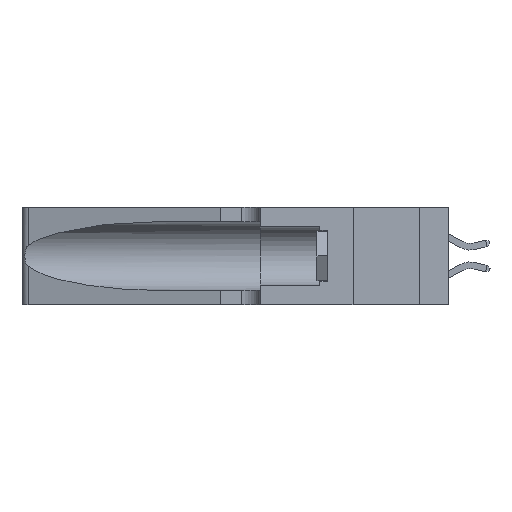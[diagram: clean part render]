
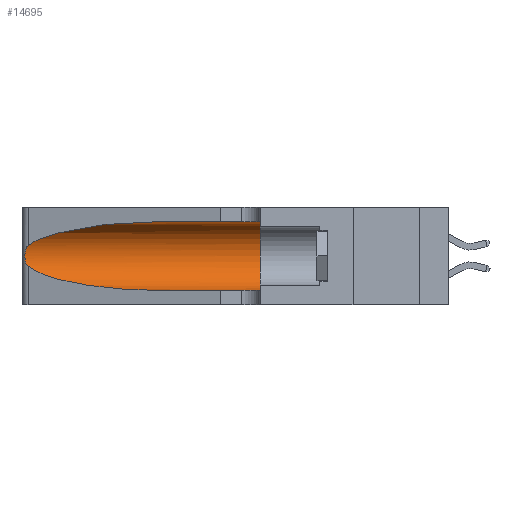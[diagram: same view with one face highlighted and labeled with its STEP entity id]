
A CAD part, left-side view. The second image highlights one B-rep face of the part: STEP entity #14695.
In plain terms, the highlighted cylindrical face has radius 3.308 mm (diameter 6.617 mm), a partial arc.
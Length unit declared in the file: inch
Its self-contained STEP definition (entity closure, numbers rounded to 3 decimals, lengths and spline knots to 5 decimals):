
#63 = VERTEX_POINT ( 'NONE', #3410 ) ;
#274 = CARTESIAN_POINT ( 'NONE',  ( 0.25789, 1.23486, 0.15765 ) ) ;
#662 = CARTESIAN_POINT ( 'NONE',  ( 0.2373, 1.15595, 0.08982 ) ) ;
#737 = CARTESIAN_POINT ( 'NONE',  ( 0.25487, 1.22718, 0.14631 ) ) ;
#1788 = CARTESIAN_POINT ( 'NONE',  ( 0.25487, 1.22718, 0.22369 ) ) ;
#1856 = CARTESIAN_POINT ( 'NONE',  ( 0.25555, 1.22993, 0.14849 ) ) ;
#2571 =( BOUNDED_CURVE ( )  B_SPLINE_CURVE ( 3, ( #16395, #17881, #8859, #19419 ),
 .UNSPECIFIED., .F., .F. ) 
 B_SPLINE_CURVE_WITH_KNOTS ( ( 4, 4 ),
 ( 1.5708, 2.84003 ),
 .UNSPECIFIED. ) 
 CURVE ( )  GEOMETRIC_REPRESENTATION_ITEM ( )  RATIONAL_B_SPLINE_CURVE ( ( 1., 0.87, 0.87, 1. ) ) 
 REPRESENTATION_ITEM ( '' )  );
#3218 = B_SPLINE_CURVE_WITH_KNOTS ( 'NONE', 3,
 ( #1788, #11126, #14113, #5010, #15631, #6554, #17138, #8082, #18642, #9629, #274, #11193, #1856, #12697 ),
 .UNSPECIFIED., .F., .F.,
 ( 4, 2, 2, 2, 2, 2, 4 ),
 ( 0., 0.00027, 0.00053, 0.00107, 0.0016, 0.00187, 0.00214 ),
 .UNSPECIFIED. ) ;
#3234 = CARTESIAN_POINT ( 'NONE',  ( 0.25487, 1.22718, 0.22369 ) ) ;
#3410 = CARTESIAN_POINT ( 'NONE',  ( 0.1305, 0.35, 0.31525 ) ) ;
#3639 = DIRECTION ( 'NONE',  ( 0., -1., 0. ) ) ;
#4037 = ORIENTED_EDGE ( 'NONE', *, *, #7615, .T. ) ;
#4151 =( BOUNDED_CURVE ( )  B_SPLINE_CURVE ( 3, ( #737, #662, #8533, #11639 ),
 .UNSPECIFIED., .F., .F. ) 
 B_SPLINE_CURVE_WITH_KNOTS ( ( 4, 4 ),
 ( 3.44316, 4.71239 ),
 .UNSPECIFIED. ) 
 CURVE ( )  GEOMETRIC_REPRESENTATION_ITEM ( )  RATIONAL_B_SPLINE_CURVE ( ( 1., 0.87, 0.87, 1. ) ) 
 REPRESENTATION_ITEM ( '' )  );
#4871 = LINE ( 'NONE', #17054, #16971 ) ;
#4933 = ORIENTED_EDGE ( 'NONE', *, *, #10686, .T. ) ;
#5001 = VERTEX_POINT ( 'NONE', #3234 ) ;
#5006 = VERTEX_POINT ( 'NONE', #16998 ) ;
#5010 = CARTESIAN_POINT ( 'NONE',  ( 0.25787, 1.23484, 0.2124 ) ) ;
#5095 = ORIENTED_EDGE ( 'NONE', *, *, #9715, .T. ) ;
#5724 = CARTESIAN_POINT ( 'NONE',  ( 0.1305, 0.35, 0.05475 ) ) ;
#5844 = AXIS2_PLACEMENT_3D ( 'NONE', #5921, #19493, #16521 ) ;
#5905 = ORIENTED_EDGE ( 'NONE', *, *, #11328, .F. ) ;
#5921 = CARTESIAN_POINT ( 'NONE',  ( 0.1305, 1.61858, 0.185 ) ) ;
#6327 = EDGE_LOOP ( 'NONE', ( #4933, #5095, #4037, #11713, #5905, #15191 ) ) ;
#6554 = CARTESIAN_POINT ( 'NONE',  ( 0.26018, 1.23835, 0.19895 ) ) ;
#6776 = CARTESIAN_POINT ( 'NONE',  ( 0.1305, 1.61858, 0.05475 ) ) ;
#6804 = CARTESIAN_POINT ( 'NONE',  ( 0.1305, 0.72297, 0.05475 ) ) ;
#6993 = CIRCLE ( 'NONE', #10850, 0.13025 ) ;
#7615 = EDGE_CURVE ( 'NONE', #13913, #9398, #4151, .T. ) ;
#7861 = CYLINDRICAL_SURFACE ( 'NONE', #5844, 0.13025 ) ;
#7997 = DIRECTION ( 'NONE',  ( 0., -1., 0. ) ) ;
#8082 = CARTESIAN_POINT ( 'NONE',  ( 0.26075, 1.23896, 0.178 ) ) ;
#8176 = EDGE_CURVE ( 'NONE', #9398, #10665, #16344, .T. ) ;
#8533 = CARTESIAN_POINT ( 'NONE',  ( 0.18966, 0.96281, 0.05475 ) ) ;
#8696 = CARTESIAN_POINT ( 'NONE',  ( 0.25487, 1.22718, 0.14631 ) ) ;
#8859 = CARTESIAN_POINT ( 'NONE',  ( 0.2373, 1.15595, 0.28018 ) ) ;
#8977 = CARTESIAN_POINT ( 'NONE',  ( 0.1305, 0.35, 0.185 ) ) ;
#9398 = VERTEX_POINT ( 'NONE', #6804 ) ;
#9629 = CARTESIAN_POINT ( 'NONE',  ( 0.25856, 1.23593, 0.16098 ) ) ;
#9715 = EDGE_CURVE ( 'NONE', #5001, #13913, #3218, .T. ) ;
#10332 = EDGE_CURVE ( 'NONE', #5006, #63, #4871, .T. ) ;
#10531 = DIRECTION ( 'NONE',  ( 0., 0., 1. ) ) ;
#10665 = VERTEX_POINT ( 'NONE', #5724 ) ;
#10686 = EDGE_CURVE ( 'NONE', #5006, #5001, #2571, .T. ) ;
#10850 = AXIS2_PLACEMENT_3D ( 'NONE', #8977, #19536, #10531 ) ;
#11126 = CARTESIAN_POINT ( 'NONE',  ( 0.25555, 1.22994, 0.2215 ) ) ;
#11193 = CARTESIAN_POINT ( 'NONE',  ( 0.25639, 1.23186, 0.15144 ) ) ;
#11328 = EDGE_CURVE ( 'NONE', #63, #10665, #6993, .T. ) ;
#11639 = CARTESIAN_POINT ( 'NONE',  ( 0.1305, 0.72297, 0.05475 ) ) ;
#11713 = ORIENTED_EDGE ( 'NONE', *, *, #8176, .T. ) ;
#12697 = CARTESIAN_POINT ( 'NONE',  ( 0.25487, 1.22718, 0.14631 ) ) ;
#13913 = VERTEX_POINT ( 'NONE', #8696 ) ;
#14113 = CARTESIAN_POINT ( 'NONE',  ( 0.25639, 1.23184, 0.21858 ) ) ;
#14695 = ADVANCED_FACE ( 'NONE', ( #15925 ), #7861, .F. ) ;
#15191 = ORIENTED_EDGE ( 'NONE', *, *, #10332, .F. ) ;
#15631 = CARTESIAN_POINT ( 'NONE',  ( 0.25854, 1.2359, 0.20912 ) ) ;
#15870 = VECTOR ( 'NONE', #3639, 39.37008 ) ;
#15925 = FACE_OUTER_BOUND ( 'NONE', #6327, .T. ) ;
#16344 = LINE ( 'NONE', #6776, #15870 ) ;
#16395 = CARTESIAN_POINT ( 'NONE',  ( 0.1305, 0.72297, 0.31525 ) ) ;
#16521 = DIRECTION ( 'NONE',  ( 0., 0., -1. ) ) ;
#16971 = VECTOR ( 'NONE', #7997, 39.37008 ) ;
#16998 = CARTESIAN_POINT ( 'NONE',  ( 0.1305, 0.72297, 0.31525 ) ) ;
#17054 = CARTESIAN_POINT ( 'NONE',  ( 0.1305, 1.61858, 0.31525 ) ) ;
#17138 = CARTESIAN_POINT ( 'NONE',  ( 0.26075, 1.23896, 0.19203 ) ) ;
#17881 = CARTESIAN_POINT ( 'NONE',  ( 0.18966, 0.96281, 0.31525 ) ) ;
#18642 = CARTESIAN_POINT ( 'NONE',  ( 0.26017, 1.23833, 0.17102 ) ) ;
#19419 = CARTESIAN_POINT ( 'NONE',  ( 0.25487, 1.22718, 0.22369 ) ) ;
#19493 = DIRECTION ( 'NONE',  ( 0., -1., 0. ) ) ;
#19536 = DIRECTION ( 'NONE',  ( 0., 1., 0. ) ) ;
